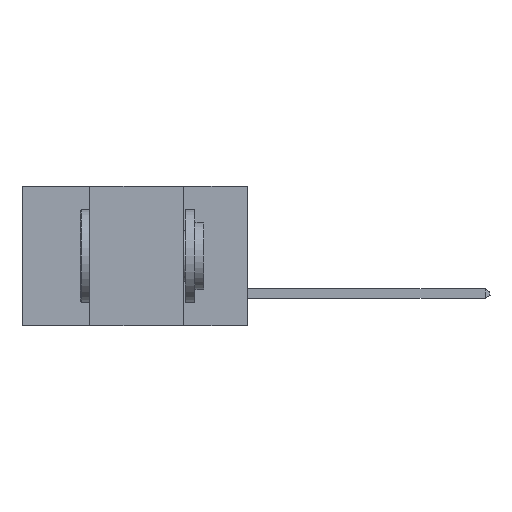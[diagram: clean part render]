
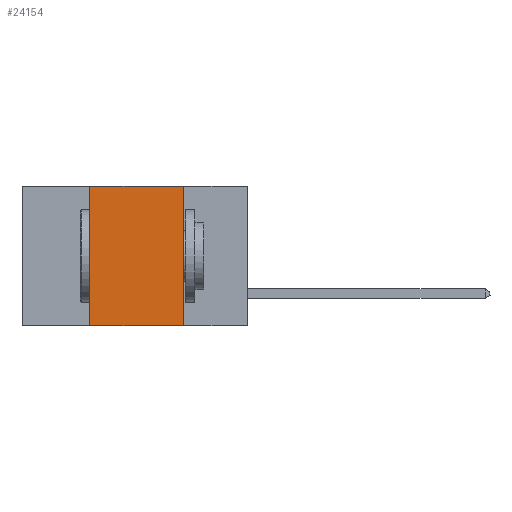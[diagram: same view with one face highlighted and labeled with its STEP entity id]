
A CAD part, left-side view. The second image highlights one B-rep face of the part: STEP entity #24154.
In plain terms, the highlighted planar face has unit normal (-1, 0, 0).
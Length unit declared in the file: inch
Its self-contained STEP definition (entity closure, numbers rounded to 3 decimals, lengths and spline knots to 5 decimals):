
#13 = LINE ( 'NONE', #7135, #28315 ) ;
#773 = DIRECTION ( 'NONE',  ( 0., 0., -1. ) ) ;
#3043 = LINE ( 'NONE', #15275, #4820 ) ;
#4820 = VECTOR ( 'NONE', #12851, 39.37008 ) ;
#7135 = CARTESIAN_POINT ( 'NONE',  ( 0., 0.6, 0. ) ) ;
#7719 = ORIENTED_EDGE ( 'NONE', *, *, #23287, .T. ) ;
#8045 = DIRECTION ( 'NONE',  ( 0., -1., 0. ) ) ;
#8713 = EDGE_CURVE ( 'NONE', #20308, #14713, #20427, .T. ) ;
#9267 = CARTESIAN_POINT ( 'NONE',  ( 0., 0.17, -0.37 ) ) ;
#10614 = CARTESIAN_POINT ( 'NONE',  ( 0., 0.17, 0. ) ) ;
#10621 = LINE ( 'NONE', #23259, #17606 ) ;
#11726 = DIRECTION ( 'NONE',  ( 0., -1., 0. ) ) ;
#12851 = DIRECTION ( 'NONE',  ( 0., 0., -1. ) ) ;
#13781 = VECTOR ( 'NONE', #21835, 39.37008 ) ;
#13887 = ORIENTED_EDGE ( 'NONE', *, *, #8713, .F. ) ;
#14713 = VERTEX_POINT ( 'NONE', #15547 ) ;
#15275 = CARTESIAN_POINT ( 'NONE',  ( 0., 0.17, 0. ) ) ;
#15302 = EDGE_CURVE ( 'NONE', #21734, #16078, #3043, .T. ) ;
#15547 = CARTESIAN_POINT ( 'NONE',  ( 0., 0.42, 0. ) ) ;
#15576 = AXIS2_PLACEMENT_3D ( 'NONE', #20411, #22650, #773 ) ;
#16078 = VERTEX_POINT ( 'NONE', #9267 ) ;
#17606 = VECTOR ( 'NONE', #8045, 39.37008 ) ;
#18170 = PLANE ( 'NONE',  #15576 ) ;
#18235 = FACE_OUTER_BOUND ( 'NONE', #19697, .T. ) ;
#19188 = ORIENTED_EDGE ( 'NONE', *, *, #15302, .F. ) ;
#19473 = CARTESIAN_POINT ( 'NONE',  ( 0., 0.42, -0.37 ) ) ;
#19697 = EDGE_LOOP ( 'NONE', ( #19188, #27919, #13887, #7719 ) ) ;
#20308 = VERTEX_POINT ( 'NONE', #19473 ) ;
#20411 = CARTESIAN_POINT ( 'NONE',  ( 0., 0.6, 0. ) ) ;
#20427 = LINE ( 'NONE', #21638, #13781 ) ;
#21638 = CARTESIAN_POINT ( 'NONE',  ( 0., 0.42, 0. ) ) ;
#21734 = VERTEX_POINT ( 'NONE', #10614 ) ;
#21835 = DIRECTION ( 'NONE',  ( 0., 0., 1. ) ) ;
#22650 = DIRECTION ( 'NONE',  ( 1., 0., 0. ) ) ;
#23259 = CARTESIAN_POINT ( 'NONE',  ( 0., 0.6, -0.37 ) ) ;
#23287 = EDGE_CURVE ( 'NONE', #20308, #16078, #10621, .T. ) ;
#24154 = ADVANCED_FACE ( 'NONE', ( #18235 ), #18170, .F. ) ;
#25718 = EDGE_CURVE ( 'NONE', #14713, #21734, #13, .T. ) ;
#27919 = ORIENTED_EDGE ( 'NONE', *, *, #25718, .F. ) ;
#28315 = VECTOR ( 'NONE', #11726, 39.37008 ) ;
